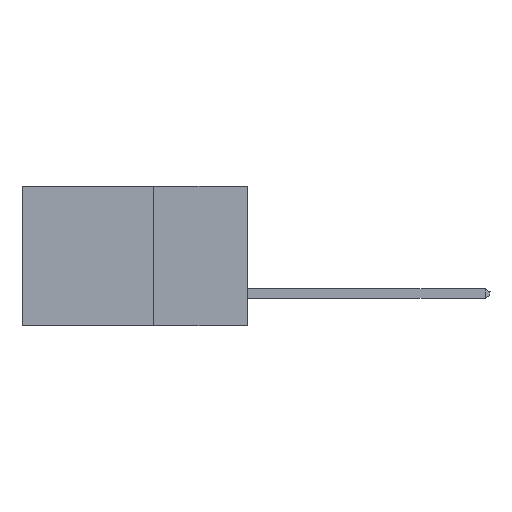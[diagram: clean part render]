
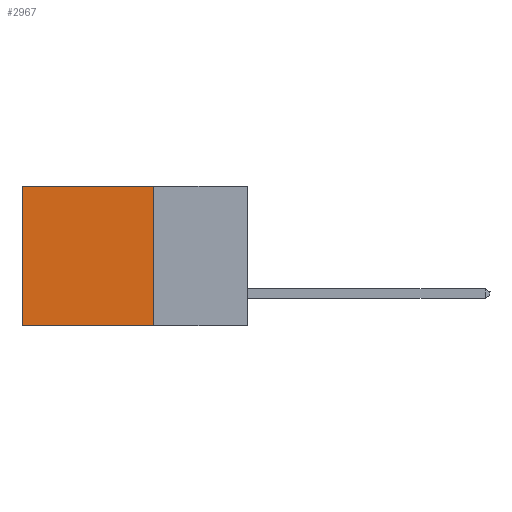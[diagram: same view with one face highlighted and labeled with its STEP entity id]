
A CAD part, left-side view. The second image highlights one B-rep face of the part: STEP entity #2967.
In plain terms, the highlighted planar face has unit normal (-1, 0, 0).
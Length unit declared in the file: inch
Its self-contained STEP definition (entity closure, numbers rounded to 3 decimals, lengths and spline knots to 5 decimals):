
#99 = DIRECTION ( 'NONE',  ( 0., 0., -1. ) ) ;
#125 = EDGE_CURVE ( 'NONE', #434, #4138, #10505, .T. ) ;
#412 = CARTESIAN_POINT ( 'NONE',  ( 0.2615, 0.25, -0.37 ) ) ;
#434 = VERTEX_POINT ( 'NONE', #10343 ) ;
#863 = CARTESIAN_POINT ( 'NONE',  ( 0.2615, 0.6, -0.37 ) ) ;
#1002 = DIRECTION ( 'NONE',  ( 1., 0., 0. ) ) ;
#1853 = VECTOR ( 'NONE', #99, 39.37008 ) ;
#2040 = AXIS2_PLACEMENT_3D ( 'NONE', #5346, #1002, #4454 ) ;
#2669 = CARTESIAN_POINT ( 'NONE',  ( 0.2615, 0.6, -0.37 ) ) ;
#2926 = ORIENTED_EDGE ( 'NONE', *, *, #6171, .T. ) ;
#2967 = ADVANCED_FACE ( 'NONE', ( #4142 ), #5294, .F. ) ;
#3477 = LINE ( 'NONE', #6940, #4123 ) ;
#3819 = ORIENTED_EDGE ( 'NONE', *, *, #125, .T. ) ;
#4123 = VECTOR ( 'NONE', #9121, 39.37008 ) ;
#4138 = VERTEX_POINT ( 'NONE', #863 ) ;
#4142 = FACE_OUTER_BOUND ( 'NONE', #10271, .T. ) ;
#4185 = VECTOR ( 'NONE', #5185, 39.37008 ) ;
#4454 = DIRECTION ( 'NONE',  ( 0., 0., -1. ) ) ;
#5185 = DIRECTION ( 'NONE',  ( 0., 0., -1. ) ) ;
#5294 = PLANE ( 'NONE',  #2040 ) ;
#5346 = CARTESIAN_POINT ( 'NONE',  ( 0.2615, 0.25, -0.37 ) ) ;
#6171 = EDGE_CURVE ( 'NONE', #9715, #434, #7734, .T. ) ;
#6757 = DIRECTION ( 'NONE',  ( 0., 1., 0. ) ) ;
#6940 = CARTESIAN_POINT ( 'NONE',  ( 0.2615, 0.25, -0.37 ) ) ;
#7244 = EDGE_CURVE ( 'NONE', #9715, #7917, #11119, .T. ) ;
#7303 = VECTOR ( 'NONE', #6757, 39.37008 ) ;
#7557 = CARTESIAN_POINT ( 'NONE',  ( 0.2615, 0.25, 0. ) ) ;
#7734 = LINE ( 'NONE', #7557, #7303 ) ;
#7858 = EDGE_CURVE ( 'NONE', #7917, #4138, #3477, .T. ) ;
#7917 = VERTEX_POINT ( 'NONE', #412 ) ;
#7936 = CARTESIAN_POINT ( 'NONE',  ( 0.2615, 0.25, -0.37 ) ) ;
#9121 = DIRECTION ( 'NONE',  ( 0., 1., 0. ) ) ;
#9715 = VERTEX_POINT ( 'NONE', #10149 ) ;
#10058 = ORIENTED_EDGE ( 'NONE', *, *, #7244, .F. ) ;
#10095 = ORIENTED_EDGE ( 'NONE', *, *, #7858, .F. ) ;
#10149 = CARTESIAN_POINT ( 'NONE',  ( 0.2615, 0.25, 0. ) ) ;
#10271 = EDGE_LOOP ( 'NONE', ( #3819, #10095, #10058, #2926 ) ) ;
#10343 = CARTESIAN_POINT ( 'NONE',  ( 0.2615, 0.6, 0. ) ) ;
#10505 = LINE ( 'NONE', #2669, #4185 ) ;
#11119 = LINE ( 'NONE', #7936, #1853 ) ;
